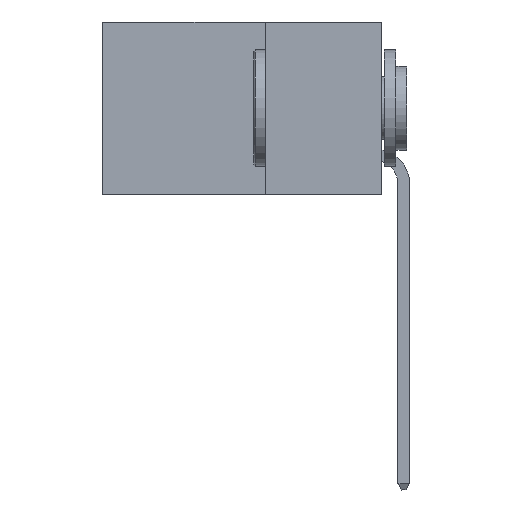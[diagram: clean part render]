
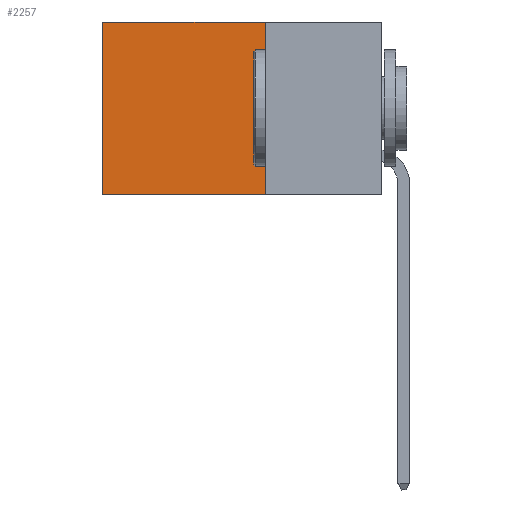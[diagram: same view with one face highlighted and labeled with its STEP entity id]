
A CAD part, left-side view. The second image highlights one B-rep face of the part: STEP entity #2257.
In plain terms, the highlighted planar face has unit normal (-1, 0, 0).
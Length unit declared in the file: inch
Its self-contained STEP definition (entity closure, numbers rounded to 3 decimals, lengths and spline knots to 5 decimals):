
#1483 = CARTESIAN_POINT ( 'NONE',  ( 0.2875, 0.25, 0. ) ) ;
#2257 = ADVANCED_FACE ( 'NONE', ( #28175 ), #15889, .F. ) ;
#2467 = DIRECTION ( 'NONE',  ( 0., 1., 0. ) ) ;
#3624 = CARTESIAN_POINT ( 'NONE',  ( 0.2875, 0.6, -0.37 ) ) ;
#4872 = LINE ( 'NONE', #28315, #9756 ) ;
#6328 = DIRECTION ( 'NONE',  ( 0., 0., -1. ) ) ;
#6995 = DIRECTION ( 'NONE',  ( 0., 1., 0. ) ) ;
#7477 = LINE ( 'NONE', #16877, #25141 ) ;
#8296 = ORIENTED_EDGE ( 'NONE', *, *, #20221, .T. ) ;
#8401 = EDGE_CURVE ( 'NONE', #27239, #14865, #4872, .T. ) ;
#8628 = LINE ( 'NONE', #20467, #20677 ) ;
#9073 = EDGE_LOOP ( 'NONE', ( #14517, #15112, #15942, #8296 ) ) ;
#9756 = VECTOR ( 'NONE', #16389, 39.37008 ) ;
#9797 = LINE ( 'NONE', #28494, #21846 ) ;
#13875 = CARTESIAN_POINT ( 'NONE',  ( 0.2875, 0.6, 0. ) ) ;
#14517 = ORIENTED_EDGE ( 'NONE', *, *, #8401, .T. ) ;
#14865 = VERTEX_POINT ( 'NONE', #3624 ) ;
#15112 = ORIENTED_EDGE ( 'NONE', *, *, #19250, .F. ) ;
#15738 = VERTEX_POINT ( 'NONE', #26239 ) ;
#15889 = PLANE ( 'NONE',  #27540 ) ;
#15942 = ORIENTED_EDGE ( 'NONE', *, *, #19939, .F. ) ;
#16389 = DIRECTION ( 'NONE',  ( 0., 0., -1. ) ) ;
#16877 = CARTESIAN_POINT ( 'NONE',  ( 0.2875, 0.25, 0. ) ) ;
#19250 = EDGE_CURVE ( 'NONE', #26531, #14865, #9797, .T. ) ;
#19939 = EDGE_CURVE ( 'NONE', #15738, #26531, #8628, .T. ) ;
#20221 = EDGE_CURVE ( 'NONE', #15738, #27239, #7477, .T. ) ;
#20467 = CARTESIAN_POINT ( 'NONE',  ( 0.2875, 0.25, 0. ) ) ;
#20677 = VECTOR ( 'NONE', #22881, 39.37008 ) ;
#20737 = DIRECTION ( 'NONE',  ( 1., 0., 0. ) ) ;
#21846 = VECTOR ( 'NONE', #6995, 39.37008 ) ;
#22881 = DIRECTION ( 'NONE',  ( 0., 0., -1. ) ) ;
#25141 = VECTOR ( 'NONE', #2467, 39.37008 ) ;
#26239 = CARTESIAN_POINT ( 'NONE',  ( 0.2875, 0.25, 0. ) ) ;
#26531 = VERTEX_POINT ( 'NONE', #28057 ) ;
#27239 = VERTEX_POINT ( 'NONE', #13875 ) ;
#27540 = AXIS2_PLACEMENT_3D ( 'NONE', #1483, #20737, #6328 ) ;
#28057 = CARTESIAN_POINT ( 'NONE',  ( 0.2875, 0.25, -0.37 ) ) ;
#28175 = FACE_OUTER_BOUND ( 'NONE', #9073, .T. ) ;
#28315 = CARTESIAN_POINT ( 'NONE',  ( 0.2875, 0.6, 0. ) ) ;
#28494 = CARTESIAN_POINT ( 'NONE',  ( 0.2875, 0.25, -0.37 ) ) ;
